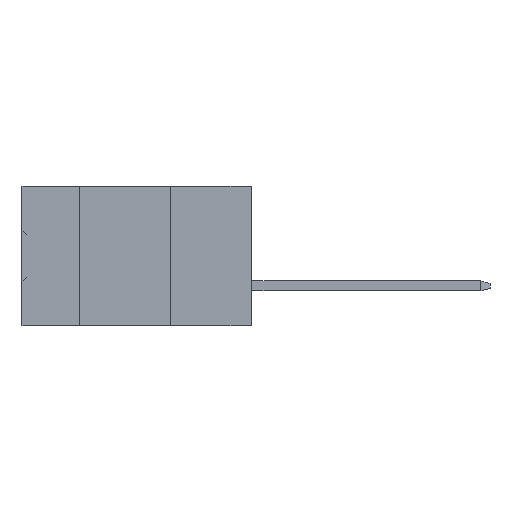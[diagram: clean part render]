
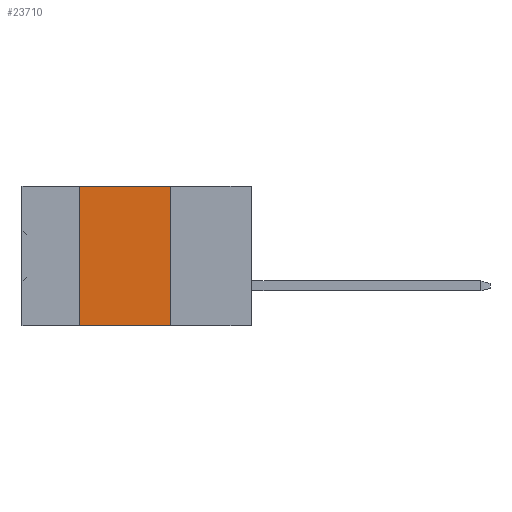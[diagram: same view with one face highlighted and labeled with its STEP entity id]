
A CAD part, left-side view. The second image highlights one B-rep face of the part: STEP entity #23710.
In plain terms, the highlighted planar face has unit normal (-1, 0, 0).
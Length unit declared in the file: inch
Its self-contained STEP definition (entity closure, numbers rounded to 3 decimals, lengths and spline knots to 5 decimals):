
#1181 = ORIENTED_EDGE ( 'NONE', *, *, #16389, .T. ) ;
#2034 = DIRECTION ( 'NONE',  ( 0., -1., 0. ) ) ;
#2789 = DIRECTION ( 'NONE',  ( 0., -1., 0. ) ) ;
#3153 = EDGE_CURVE ( 'NONE', #15741, #5156, #10695, .T. ) ;
#4343 = LINE ( 'NONE', #24075, #25016 ) ;
#5156 = VERTEX_POINT ( 'NONE', #11339 ) ;
#6217 = VECTOR ( 'NONE', #2789, 39.37008 ) ;
#9318 = CARTESIAN_POINT ( 'NONE',  ( 0., 0.254, 0. ) ) ;
#9807 = CARTESIAN_POINT ( 'NONE',  ( 0., 0.72, -0.437 ) ) ;
#9812 = AXIS2_PLACEMENT_3D ( 'NONE', #18380, #15943, #25871 ) ;
#9895 = VERTEX_POINT ( 'NONE', #18541 ) ;
#10052 = ORIENTED_EDGE ( 'NONE', *, *, #26549, .F. ) ;
#10408 = DIRECTION ( 'NONE',  ( 0., 0., -1. ) ) ;
#10695 = LINE ( 'NONE', #10851, #28643 ) ;
#10724 = LINE ( 'NONE', #30143, #26573 ) ;
#10851 = CARTESIAN_POINT ( 'NONE',  ( 0., 0.54, -0.437 ) ) ;
#11339 = CARTESIAN_POINT ( 'NONE',  ( 0., 0.54, 0. ) ) ;
#12010 = VERTEX_POINT ( 'NONE', #9318 ) ;
#13615 = EDGE_LOOP ( 'NONE', ( #16017, #10052, #17359, #1181 ) ) ;
#15741 = VERTEX_POINT ( 'NONE', #18366 ) ;
#15943 = DIRECTION ( 'NONE',  ( 1., 0., 0. ) ) ;
#16017 = ORIENTED_EDGE ( 'NONE', *, *, #16933, .F. ) ;
#16073 = DIRECTION ( 'NONE',  ( 0., 0., 1. ) ) ;
#16389 = EDGE_CURVE ( 'NONE', #15741, #9895, #25143, .T. ) ;
#16933 = EDGE_CURVE ( 'NONE', #12010, #9895, #10724, .T. ) ;
#17359 = ORIENTED_EDGE ( 'NONE', *, *, #3153, .F. ) ;
#18220 = FACE_OUTER_BOUND ( 'NONE', #13615, .T. ) ;
#18366 = CARTESIAN_POINT ( 'NONE',  ( 0., 0.54, -0.437 ) ) ;
#18380 = CARTESIAN_POINT ( 'NONE',  ( 0., 0.72, 0. ) ) ;
#18541 = CARTESIAN_POINT ( 'NONE',  ( 0., 0.254, -0.437 ) ) ;
#23710 = ADVANCED_FACE ( 'NONE', ( #18220 ), #28152, .F. ) ;
#24075 = CARTESIAN_POINT ( 'NONE',  ( 0., 0.72, 0. ) ) ;
#25016 = VECTOR ( 'NONE', #2034, 39.37008 ) ;
#25143 = LINE ( 'NONE', #9807, #6217 ) ;
#25871 = DIRECTION ( 'NONE',  ( 0., 0., -1. ) ) ;
#26549 = EDGE_CURVE ( 'NONE', #5156, #12010, #4343, .T. ) ;
#26573 = VECTOR ( 'NONE', #10408, 39.37008 ) ;
#28152 = PLANE ( 'NONE',  #9812 ) ;
#28643 = VECTOR ( 'NONE', #16073, 39.37008 ) ;
#30143 = CARTESIAN_POINT ( 'NONE',  ( 0., 0.254, -0.437 ) ) ;
